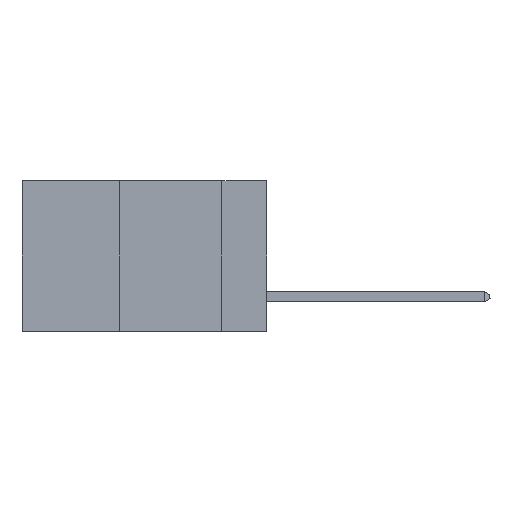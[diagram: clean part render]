
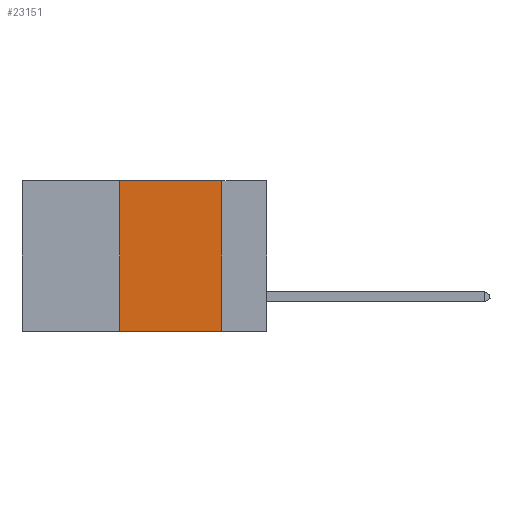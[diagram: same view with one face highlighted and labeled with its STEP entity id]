
A CAD part, left-side view. The second image highlights one B-rep face of the part: STEP entity #23151.
In plain terms, the highlighted planar face has unit normal (-1, 0, 0).
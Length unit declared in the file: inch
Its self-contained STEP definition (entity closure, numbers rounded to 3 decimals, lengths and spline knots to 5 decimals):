
#106 = CARTESIAN_POINT ( 'NONE',  ( 0., 0.11, -0.37 ) ) ;
#865 = ORIENTED_EDGE ( 'NONE', *, *, #36446, .F. ) ;
#1024 = LINE ( 'NONE', #5270, #21718 ) ;
#1794 = VERTEX_POINT ( 'NONE', #33380 ) ;
#2257 = CARTESIAN_POINT ( 'NONE',  ( 0., 0.36, 0. ) ) ;
#5270 = CARTESIAN_POINT ( 'NONE',  ( 0., 0.11, 0. ) ) ;
#6563 = VECTOR ( 'NONE', #6867, 39.37008 ) ;
#6817 = VERTEX_POINT ( 'NONE', #106 ) ;
#6867 = DIRECTION ( 'NONE',  ( 0., -1., 0. ) ) ;
#8924 = LINE ( 'NONE', #2257, #32688 ) ;
#12831 = DIRECTION ( 'NONE',  ( 0., -1., 0. ) ) ;
#13194 = DIRECTION ( 'NONE',  ( 0., 0., 1. ) ) ;
#15337 = EDGE_CURVE ( 'NONE', #21244, #6817, #40421, .T. ) ;
#17159 = EDGE_CURVE ( 'NONE', #1794, #6817, #1024, .T. ) ;
#17468 = ORIENTED_EDGE ( 'NONE', *, *, #17159, .F. ) ;
#17912 = PLANE ( 'NONE',  #33838 ) ;
#20292 = DIRECTION ( 'NONE',  ( 0., 0., -1. ) ) ;
#20953 = VERTEX_POINT ( 'NONE', #33893 ) ;
#21244 = VERTEX_POINT ( 'NONE', #35203 ) ;
#21718 = VECTOR ( 'NONE', #20292, 39.37008 ) ;
#23081 = EDGE_LOOP ( 'NONE', ( #17468, #32842, #865, #48334 ) ) ;
#23151 = ADVANCED_FACE ( 'NONE', ( #32997 ), #17912, .F. ) ;
#29647 = EDGE_CURVE ( 'NONE', #20953, #1794, #31981, .T. ) ;
#30180 = VECTOR ( 'NONE', #12831, 39.37008 ) ;
#31981 = LINE ( 'NONE', #35584, #30180 ) ;
#32688 = VECTOR ( 'NONE', #13194, 39.37008 ) ;
#32842 = ORIENTED_EDGE ( 'NONE', *, *, #29647, .F. ) ;
#32997 = FACE_OUTER_BOUND ( 'NONE', #23081, .T. ) ;
#33380 = CARTESIAN_POINT ( 'NONE',  ( 0., 0.11, 0. ) ) ;
#33838 = AXIS2_PLACEMENT_3D ( 'NONE', #41014, #36563, #44693 ) ;
#33893 = CARTESIAN_POINT ( 'NONE',  ( 0., 0.36, 0. ) ) ;
#35203 = CARTESIAN_POINT ( 'NONE',  ( 0., 0.36, -0.37 ) ) ;
#35584 = CARTESIAN_POINT ( 'NONE',  ( 0., 0.6, 0. ) ) ;
#36446 = EDGE_CURVE ( 'NONE', #21244, #20953, #8924, .T. ) ;
#36563 = DIRECTION ( 'NONE',  ( 1., 0., 0. ) ) ;
#36914 = CARTESIAN_POINT ( 'NONE',  ( 0., 0.6, -0.37 ) ) ;
#40421 = LINE ( 'NONE', #36914, #6563 ) ;
#41014 = CARTESIAN_POINT ( 'NONE',  ( 0., 0.6, 0. ) ) ;
#44693 = DIRECTION ( 'NONE',  ( 0., 0., -1. ) ) ;
#48334 = ORIENTED_EDGE ( 'NONE', *, *, #15337, .T. ) ;
